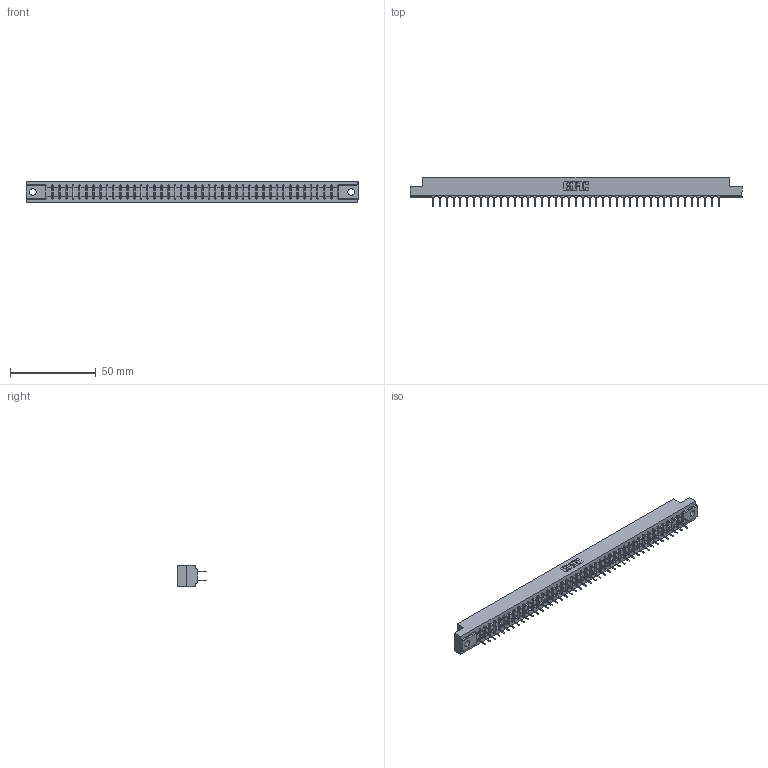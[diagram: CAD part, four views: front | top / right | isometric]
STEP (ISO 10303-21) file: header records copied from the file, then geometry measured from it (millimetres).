
FILE_DESCRIPTION (( 'STEP AP203' ), '1' );
FILE_NAME ('357-086-524-204.STEP', '2019-09-19T18:59:38', ( '' ), ( '' ), 'SwSTEP 2.0', 'SolidWorks 2016', '' );
FILE_SCHEMA (( 'CONFIG_CONTROL_DESIGN' ));
Length unit declared in the file: inch
Products named in the file (3): 357-086-524-204; 307-290-001_524; 307 Part_.156 Dia Mounting Holes
Assembly tree (87 placements, depth 2):
  357-086-524-204
    307 Part_.156 Dia Mounting Holes
    307-290-001_524  x86
Bounding box: 193.4 x 17.42 x 12.7 mm (x, y, z)
Volume: 20438.7 mm3; surface area: 24567.7 mm2
Topology: 87 solids, 87 shells, 4132 faces, 11539 edges, 7458 vertices
Faces by surface type: plane 2750, cylinder 1294, sphere 88
Entity records: 38502 total; most frequent: CARTESIAN_POINT 6301, ORIENTED_EDGE 6242, DIRECTION 6163, EDGE_CURVE 3121, LINE 2403, VECTOR 2403, VERTEX_POINT 2018, AXIS2_PLACEMENT_3D 1880
